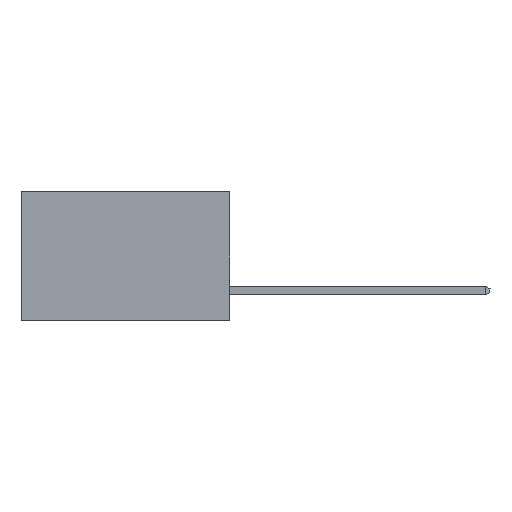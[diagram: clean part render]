
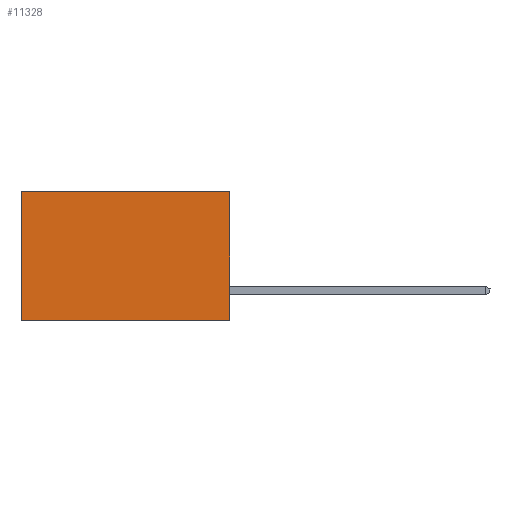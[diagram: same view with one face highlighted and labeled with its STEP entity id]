
A CAD part, left-side view. The second image highlights one B-rep face of the part: STEP entity #11328.
In plain terms, the highlighted planar face has unit normal (-1, 0, 0).
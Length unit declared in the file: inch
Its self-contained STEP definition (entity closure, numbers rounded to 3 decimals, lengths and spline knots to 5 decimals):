
#157 = CARTESIAN_POINT ( 'NONE',  ( 0.2615, 0.6, 0. ) ) ;
#749 = LINE ( 'NONE', #1924, #793 ) ;
#793 = VECTOR ( 'NONE', #4011, 39.37008 ) ;
#947 = VECTOR ( 'NONE', #7576, 39.37008 ) ;
#1325 = CARTESIAN_POINT ( 'NONE',  ( 0.2615, 0., -0.37 ) ) ;
#1924 = CARTESIAN_POINT ( 'NONE',  ( 0.2615, 0.6, -0.37 ) ) ;
#2479 = ORIENTED_EDGE ( 'NONE', *, *, #13766, .F. ) ;
#3457 = EDGE_LOOP ( 'NONE', ( #9937, #2479, #12340, #7534 ) ) ;
#3672 = CARTESIAN_POINT ( 'NONE',  ( 0.2615, 0., -0.37 ) ) ;
#4011 = DIRECTION ( 'NONE',  ( 0., 0., -1. ) ) ;
#4311 = CARTESIAN_POINT ( 'NONE',  ( 0.2615, 0., -0.37 ) ) ;
#4573 = EDGE_CURVE ( 'NONE', #11786, #4819, #749, .T. ) ;
#4672 = VECTOR ( 'NONE', #11326, 39.37008 ) ;
#4819 = VERTEX_POINT ( 'NONE', #11338 ) ;
#5158 = VECTOR ( 'NONE', #6343, 39.37008 ) ;
#5310 = AXIS2_PLACEMENT_3D ( 'NONE', #9831, #7747, #11222 ) ;
#5713 = PLANE ( 'NONE',  #5310 ) ;
#6343 = DIRECTION ( 'NONE',  ( 0., 1., 0. ) ) ;
#7452 = VERTEX_POINT ( 'NONE', #3672 ) ;
#7534 = ORIENTED_EDGE ( 'NONE', *, *, #8116, .T. ) ;
#7576 = DIRECTION ( 'NONE',  ( 0., 1., 0. ) ) ;
#7747 = DIRECTION ( 'NONE',  ( 1., 0., 0. ) ) ;
#8116 = EDGE_CURVE ( 'NONE', #9571, #11786, #11905, .T. ) ;
#9571 = VERTEX_POINT ( 'NONE', #11079 ) ;
#9831 = CARTESIAN_POINT ( 'NONE',  ( 0.2615, 0., -0.37 ) ) ;
#9908 = FACE_OUTER_BOUND ( 'NONE', #3457, .T. ) ;
#9937 = ORIENTED_EDGE ( 'NONE', *, *, #4573, .T. ) ;
#11079 = CARTESIAN_POINT ( 'NONE',  ( 0.2615, 0., 0. ) ) ;
#11222 = DIRECTION ( 'NONE',  ( 0., 0., -1. ) ) ;
#11326 = DIRECTION ( 'NONE',  ( 0., 0., -1. ) ) ;
#11328 = ADVANCED_FACE ( 'NONE', ( #9908 ), #5713, .F. ) ;
#11338 = CARTESIAN_POINT ( 'NONE',  ( 0.2615, 0.6, -0.37 ) ) ;
#11786 = VERTEX_POINT ( 'NONE', #157 ) ;
#11905 = LINE ( 'NONE', #13057, #5158 ) ;
#12070 = LINE ( 'NONE', #4311, #947 ) ;
#12259 = LINE ( 'NONE', #1325, #4672 ) ;
#12340 = ORIENTED_EDGE ( 'NONE', *, *, #14256, .F. ) ;
#13057 = CARTESIAN_POINT ( 'NONE',  ( 0.2615, 0., 0. ) ) ;
#13766 = EDGE_CURVE ( 'NONE', #7452, #4819, #12070, .T. ) ;
#14256 = EDGE_CURVE ( 'NONE', #9571, #7452, #12259, .T. ) ;
